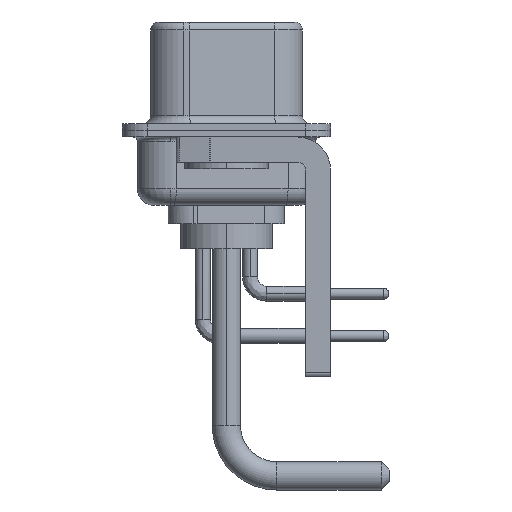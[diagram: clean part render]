
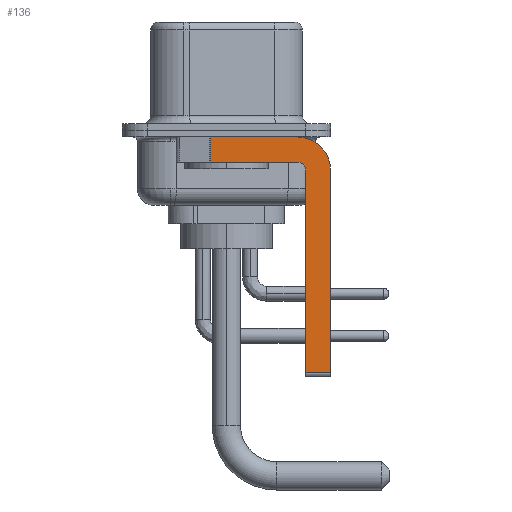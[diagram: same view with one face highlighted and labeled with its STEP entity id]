
A CAD part, left-side view. The second image highlights one B-rep face of the part: STEP entity #136.
In plain terms, the highlighted planar face has unit normal (-1, 0, 0).
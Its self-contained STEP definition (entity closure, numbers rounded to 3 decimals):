
#136 = ADVANCED_FACE ( 'NONE', ( #7205 ), #22197, .F. ) ;
#878 = ORIENTED_EDGE ( 'NONE', *, *, #17380, .F. ) ;
#1082 = VERTEX_POINT ( 'NONE', #21248 ) ;
#1399 = LINE ( 'NONE', #22311, #13443 ) ;
#1805 = CARTESIAN_POINT ( 'NONE',  ( -2.9, 0.978, -1.9 ) ) ;
#1927 = DIRECTION ( 'NONE',  ( 0., 0., -1. ) ) ;
#2191 = DIRECTION ( 'NONE',  ( 0., -1., 0. ) ) ;
#2755 = VECTOR ( 'NONE', #17634, 1000. ) ;
#3048 = EDGE_CURVE ( 'NONE', #7122, #13651, #22303, .T. ) ;
#3724 = AXIS2_PLACEMENT_3D ( 'NONE', #13233, #5351, #20604 ) ;
#5230 = DIRECTION ( 'NONE',  ( 0., 0., -1. ) ) ;
#5351 = DIRECTION ( 'NONE',  ( -1., 0., 0. ) ) ;
#5594 = CARTESIAN_POINT ( 'NONE',  ( -2.9, -4.25, -1.9 ) ) ;
#5818 = EDGE_CURVE ( 'NONE', #12403, #22424, #15223, .T. ) ;
#5888 = CARTESIAN_POINT ( 'NONE',  ( -2.9, -4.25, -14.55 ) ) ;
#6236 = CARTESIAN_POINT ( 'NONE',  ( -2.9, 0.978, -0.4 ) ) ;
#6296 = EDGE_CURVE ( 'NONE', #12403, #1082, #22820, .T. ) ;
#7122 = VERTEX_POINT ( 'NONE', #22768 ) ;
#7205 = FACE_OUTER_BOUND ( 'NONE', #12854, .T. ) ;
#7333 = VERTEX_POINT ( 'NONE', #1805 ) ;
#7405 = EDGE_CURVE ( 'NONE', #19354, #7333, #11264, .T. ) ;
#7453 = CARTESIAN_POINT ( 'NONE',  ( -2.9, -4.25, -1.9 ) ) ;
#7881 = ORIENTED_EDGE ( 'NONE', *, *, #3048, .F. ) ;
#8611 = ORIENTED_EDGE ( 'NONE', *, *, #22270, .F. ) ;
#8666 = ORIENTED_EDGE ( 'NONE', *, *, #13664, .F. ) ;
#8690 = VECTOR ( 'NONE', #15062, 1000. ) ;
#10763 = CARTESIAN_POINT ( 'NONE',  ( -2.9, -4.25, -2.4 ) ) ;
#11264 = LINE ( 'NONE', #18411, #19654 ) ;
#11788 = VECTOR ( 'NONE', #23066, 1000. ) ;
#12403 = VERTEX_POINT ( 'NONE', #15167 ) ;
#12854 = EDGE_LOOP ( 'NONE', ( #8666, #15625, #878, #8611, #17073, #13207, #14612, #7881 ) ) ;
#12973 = DIRECTION ( 'NONE',  ( 0., -1., 0. ) ) ;
#13207 = ORIENTED_EDGE ( 'NONE', *, *, #5818, .T. ) ;
#13233 = CARTESIAN_POINT ( 'NONE',  ( -2.9, -4.25, -2.4 ) ) ;
#13443 = VECTOR ( 'NONE', #12973, 1000. ) ;
#13480 = CARTESIAN_POINT ( 'NONE',  ( -2.9, -4.75, -14.8 ) ) ;
#13651 = VERTEX_POINT ( 'NONE', #16788 ) ;
#13664 = EDGE_CURVE ( 'NONE', #19354, #7122, #1399, .T. ) ;
#14612 = ORIENTED_EDGE ( 'NONE', *, *, #16461, .F. ) ;
#14944 = LINE ( 'NONE', #7453, #8690 ) ;
#15062 = DIRECTION ( 'NONE',  ( 0., 1., 0. ) ) ;
#15167 = CARTESIAN_POINT ( 'NONE',  ( -2.9, -4.75, -14.55 ) ) ;
#15223 = LINE ( 'NONE', #5888, #20005 ) ;
#15625 = ORIENTED_EDGE ( 'NONE', *, *, #7405, .T. ) ;
#15763 = CARTESIAN_POINT ( 'NONE',  ( -2.9, -6.25, -2.4 ) ) ;
#16461 = EDGE_CURVE ( 'NONE', #13651, #22424, #19947, .T. ) ;
#16788 = CARTESIAN_POINT ( 'NONE',  ( -2.9, -6.25, -2.4 ) ) ;
#17073 = ORIENTED_EDGE ( 'NONE', *, *, #6296, .F. ) ;
#17283 = CARTESIAN_POINT ( 'NONE',  ( -2.9, -6.25, -14.55 ) ) ;
#17380 = EDGE_CURVE ( 'NONE', #23241, #7333, #14944, .T. ) ;
#17634 = DIRECTION ( 'NONE',  ( 0., 0., -1. ) ) ;
#18411 = CARTESIAN_POINT ( 'NONE',  ( -2.9, 0.978, -1.9 ) ) ;
#19354 = VERTEX_POINT ( 'NONE', #6236 ) ;
#19654 = VECTOR ( 'NONE', #1927, 1000. ) ;
#19947 = LINE ( 'NONE', #15763, #2755 ) ;
#20005 = VECTOR ( 'NONE', #2191, 1000. ) ;
#20085 = CARTESIAN_POINT ( 'NONE',  ( -2.9, -4.25, -2.4 ) ) ;
#20604 = DIRECTION ( 'NONE',  ( 0., 0., 1. ) ) ;
#21008 = AXIS2_PLACEMENT_3D ( 'NONE', #10763, #23941, #5230 ) ;
#21248 = CARTESIAN_POINT ( 'NONE',  ( -2.9, -4.75, -2.4 ) ) ;
#21581 = DIRECTION ( 'NONE',  ( 1., 0., 0. ) ) ;
#22197 = PLANE ( 'NONE',  #21008 ) ;
#22270 = EDGE_CURVE ( 'NONE', #1082, #23241, #22975, .T. ) ;
#22303 = CIRCLE ( 'NONE', #23477, 2. ) ;
#22311 = CARTESIAN_POINT ( 'NONE',  ( -2.9, 3., -0.4 ) ) ;
#22424 = VERTEX_POINT ( 'NONE', #17283 ) ;
#22768 = CARTESIAN_POINT ( 'NONE',  ( -2.9, -4.25, -0.4 ) ) ;
#22820 = LINE ( 'NONE', #13480, #11788 ) ;
#22975 = CIRCLE ( 'NONE', #3724, 0.5 ) ;
#23066 = DIRECTION ( 'NONE',  ( 0., 0., 1. ) ) ;
#23241 = VERTEX_POINT ( 'NONE', #5594 ) ;
#23477 = AXIS2_PLACEMENT_3D ( 'NONE', #20085, #21581, #23794 ) ;
#23794 = DIRECTION ( 'NONE',  ( 0., 0., -1. ) ) ;
#23941 = DIRECTION ( 'NONE',  ( 1., 0., 0. ) ) ;
